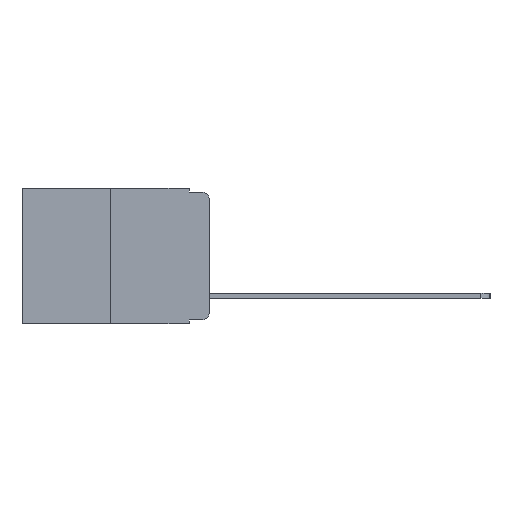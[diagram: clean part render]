
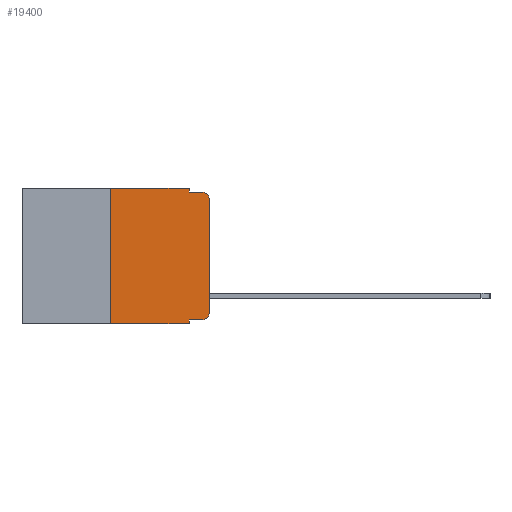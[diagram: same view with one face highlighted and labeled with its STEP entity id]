
A CAD part, left-side view. The second image highlights one B-rep face of the part: STEP entity #19400.
In plain terms, the highlighted planar face has unit normal (-1, 0, 0).
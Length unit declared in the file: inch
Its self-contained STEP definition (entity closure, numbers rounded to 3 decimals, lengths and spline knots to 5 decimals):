
#70 = ORIENTED_EDGE ( 'NONE', *, *, #2360, .F. ) ;
#74 = AXIS2_PLACEMENT_3D ( 'NONE', #2911, #3791, #2679 ) ;
#488 = DIRECTION ( 'NONE',  ( 0., 0., -1. ) ) ;
#577 = EDGE_CURVE ( 'NONE', #5439, #12273, #21670, .T. ) ;
#1038 = VERTEX_POINT ( 'NONE', #8005 ) ;
#1270 = VERTEX_POINT ( 'NONE', #13273 ) ;
#1384 = EDGE_CURVE ( 'NONE', #1270, #5887, #13173, .T. ) ;
#1610 = CARTESIAN_POINT ( 'NONE',  ( 0., 0., 0. ) ) ;
#1788 = ORIENTED_EDGE ( 'NONE', *, *, #577, .F. ) ;
#2092 = AXIS2_PLACEMENT_3D ( 'NONE', #9227, #22821, #11196 ) ;
#2095 = VECTOR ( 'NONE', #20495, 39.37008 ) ;
#2360 = EDGE_CURVE ( 'NONE', #4884, #14074, #4871, .T. ) ;
#2674 = FACE_OUTER_BOUND ( 'NONE', #21131, .T. ) ;
#2679 = DIRECTION ( 'NONE',  ( 0., 0., -1. ) ) ;
#2729 = VECTOR ( 'NONE', #5686, 39.37008 ) ;
#2911 = CARTESIAN_POINT ( 'NONE',  ( 0., 0.02, -0.313 ) ) ;
#2917 = CARTESIAN_POINT ( 'NONE',  ( 0., 0.051, -0.01 ) ) ;
#3253 = CARTESIAN_POINT ( 'NONE',  ( 0., 0., -0.313 ) ) ;
#3575 = DIRECTION ( 'NONE',  ( 0., 0., 1. ) ) ;
#3690 = CARTESIAN_POINT ( 'NONE',  ( 0., 0.473, 0. ) ) ;
#3791 = DIRECTION ( 'NONE',  ( -1., 0., 0. ) ) ;
#4231 = DIRECTION ( 'NONE',  ( 0., 0., -1. ) ) ;
#4871 = LINE ( 'NONE', #18536, #14615 ) ;
#4884 = VERTEX_POINT ( 'NONE', #19455 ) ;
#4923 = CARTESIAN_POINT ( 'NONE',  ( 0., 0., -0.03 ) ) ;
#5175 = LINE ( 'NONE', #22982, #20039 ) ;
#5219 = VERTEX_POINT ( 'NONE', #22500 ) ;
#5439 = VERTEX_POINT ( 'NONE', #11478 ) ;
#5684 = CARTESIAN_POINT ( 'NONE',  ( 0., 0.051, -0.333 ) ) ;
#5686 = DIRECTION ( 'NONE',  ( 0., -1., 0. ) ) ;
#5887 = VERTEX_POINT ( 'NONE', #3253 ) ;
#5981 = EDGE_CURVE ( 'NONE', #1038, #5219, #5175, .T. ) ;
#7240 = LINE ( 'NONE', #12002, #16966 ) ;
#7627 = DIRECTION ( 'NONE',  ( 0., -1., 0. ) ) ;
#8005 = CARTESIAN_POINT ( 'NONE',  ( 0., 0.051, -0.333 ) ) ;
#8130 = ORIENTED_EDGE ( 'NONE', *, *, #13035, .T. ) ;
#8254 = CARTESIAN_POINT ( 'NONE',  ( 0., 0.473, 0. ) ) ;
#8973 = ORIENTED_EDGE ( 'NONE', *, *, #5981, .F. ) ;
#9227 = CARTESIAN_POINT ( 'NONE',  ( 0., 0.02, -0.03 ) ) ;
#9386 = DIRECTION ( 'NONE',  ( 0., 0., -1. ) ) ;
#10463 = ORIENTED_EDGE ( 'NONE', *, *, #13650, .T. ) ;
#10826 = CARTESIAN_POINT ( 'NONE',  ( 0., 0.473, -0.343 ) ) ;
#11196 = DIRECTION ( 'NONE',  ( 0., 0., -1. ) ) ;
#11478 = CARTESIAN_POINT ( 'NONE',  ( 0., 0.051, -0.01 ) ) ;
#11844 = VECTOR ( 'NONE', #7627, 39.37008 ) ;
#12002 = CARTESIAN_POINT ( 'NONE',  ( 0., 0.051, 0. ) ) ;
#12206 = DIRECTION ( 'NONE',  ( 1., 0., 0. ) ) ;
#12273 = VERTEX_POINT ( 'NONE', #12497 ) ;
#12356 = DIRECTION ( 'NONE',  ( 0., -1., 0. ) ) ;
#12497 = CARTESIAN_POINT ( 'NONE',  ( 0., 0.02, -0.01 ) ) ;
#12530 = AXIS2_PLACEMENT_3D ( 'NONE', #8254, #12206, #488 ) ;
#12707 = CARTESIAN_POINT ( 'NONE',  ( 0., 0.25, 0. ) ) ;
#13035 = EDGE_CURVE ( 'NONE', #1038, #1270, #16976, .T. ) ;
#13173 = CIRCLE ( 'NONE', #74, 0.02 ) ;
#13273 = CARTESIAN_POINT ( 'NONE',  ( 0., 0.02, -0.333 ) ) ;
#13650 = EDGE_CURVE ( 'NONE', #5887, #17103, #18475, .T. ) ;
#14074 = VERTEX_POINT ( 'NONE', #12707 ) ;
#14159 = VERTEX_POINT ( 'NONE', #24704 ) ;
#14615 = VECTOR ( 'NONE', #17574, 39.37008 ) ;
#14770 = EDGE_CURVE ( 'NONE', #17103, #12273, #22037, .T. ) ;
#15891 = ORIENTED_EDGE ( 'NONE', *, *, #18984, .T. ) ;
#16966 = VECTOR ( 'NONE', #4231, 39.37008 ) ;
#16976 = LINE ( 'NONE', #5684, #11844 ) ;
#17103 = VERTEX_POINT ( 'NONE', #4923 ) ;
#17574 = DIRECTION ( 'NONE',  ( 0., 0., 1. ) ) ;
#17630 = LINE ( 'NONE', #10826, #2095 ) ;
#18475 = LINE ( 'NONE', #1610, #23020 ) ;
#18536 = CARTESIAN_POINT ( 'NONE',  ( 0., 0.25, 0. ) ) ;
#18549 = EDGE_CURVE ( 'NONE', #14074, #14159, #22193, .T. ) ;
#18738 = ORIENTED_EDGE ( 'NONE', *, *, #1384, .T. ) ;
#18984 = EDGE_CURVE ( 'NONE', #4884, #5219, #17630, .T. ) ;
#19175 = ORIENTED_EDGE ( 'NONE', *, *, #18549, .F. ) ;
#19400 = ADVANCED_FACE ( 'NONE', ( #2674 ), #23779, .F. ) ;
#19455 = CARTESIAN_POINT ( 'NONE',  ( 0., 0.25, -0.343 ) ) ;
#20039 = VECTOR ( 'NONE', #9386, 39.37008 ) ;
#20318 = ORIENTED_EDGE ( 'NONE', *, *, #24177, .F. ) ;
#20495 = DIRECTION ( 'NONE',  ( 0., -1., 0. ) ) ;
#20824 = ORIENTED_EDGE ( 'NONE', *, *, #14770, .T. ) ;
#21131 = EDGE_LOOP ( 'NONE', ( #10463, #20824, #1788, #20318, #19175, #70, #15891, #8973, #8130, #18738 ) ) ;
#21670 = LINE ( 'NONE', #2917, #22275 ) ;
#22037 = CIRCLE ( 'NONE', #2092, 0.02 ) ;
#22193 = LINE ( 'NONE', #3690, #2729 ) ;
#22275 = VECTOR ( 'NONE', #12356, 39.37008 ) ;
#22500 = CARTESIAN_POINT ( 'NONE',  ( 0., 0.051, -0.343 ) ) ;
#22821 = DIRECTION ( 'NONE',  ( -1., 0., 0. ) ) ;
#22982 = CARTESIAN_POINT ( 'NONE',  ( 0., 0.051, 0. ) ) ;
#23020 = VECTOR ( 'NONE', #3575, 39.37008 ) ;
#23779 = PLANE ( 'NONE',  #12530 ) ;
#24177 = EDGE_CURVE ( 'NONE', #14159, #5439, #7240, .T. ) ;
#24704 = CARTESIAN_POINT ( 'NONE',  ( 0., 0.051, 0. ) ) ;
